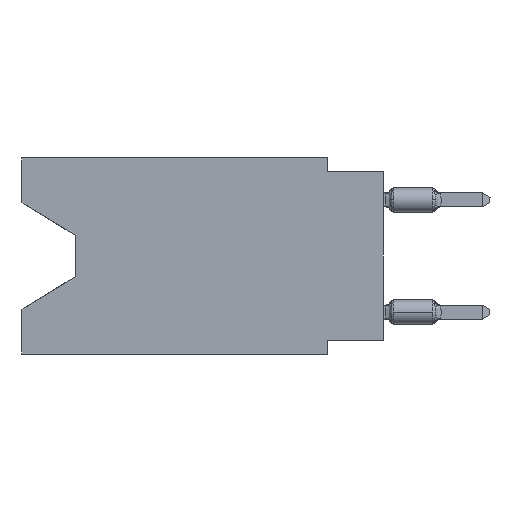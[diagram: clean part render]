
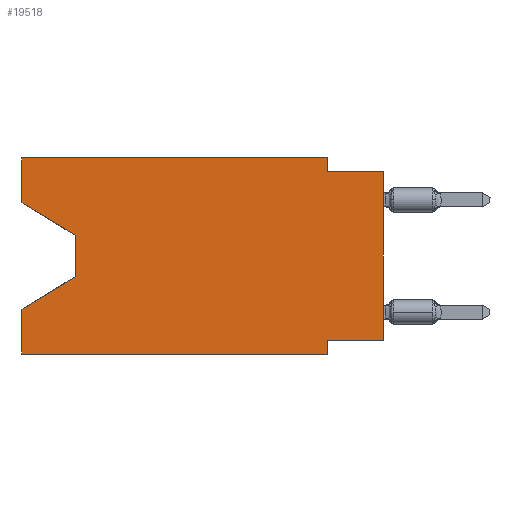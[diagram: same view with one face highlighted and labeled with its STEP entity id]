
A CAD part, left-side view. The second image highlights one B-rep face of the part: STEP entity #19518.
In plain terms, the highlighted planar face has unit normal (-1, 0, 0).
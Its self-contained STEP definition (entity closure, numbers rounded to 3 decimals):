
#23 = CARTESIAN_POINT ( 'NONE',  ( 0., 0., -0.635 ) ) ;
#571 = ORIENTED_EDGE ( 'NONE', *, *, #31390, .T. ) ;
#642 = FACE_OUTER_BOUND ( 'NONE', #12279, .T. ) ;
#667 = LINE ( 'NONE', #24504, #34688 ) ;
#1643 = VECTOR ( 'NONE', #34001, 1000. ) ;
#1932 = EDGE_CURVE ( 'NONE', #30288, #29172, #25603, .T. ) ;
#2011 = CARTESIAN_POINT ( 'NONE',  ( 0., 2.54, -8.255 ) ) ;
#3299 = CARTESIAN_POINT ( 'NONE',  ( 0., 16.383, 0. ) ) ;
#3633 = CARTESIAN_POINT ( 'NONE',  ( 0., 0., -8.255 ) ) ;
#3730 = LINE ( 'NONE', #3299, #38355 ) ;
#4187 = LINE ( 'NONE', #28236, #7925 ) ;
#4588 = CARTESIAN_POINT ( 'NONE',  ( 0., 16.383, -2.038 ) ) ;
#5256 = CARTESIAN_POINT ( 'NONE',  ( 0., 2.54, 0. ) ) ;
#6127 = VECTOR ( 'NONE', #27879, 1000. ) ;
#6147 = EDGE_CURVE ( 'NONE', #29172, #32977, #4187, .T. ) ;
#6573 = LINE ( 'NONE', #20278, #1643 ) ;
#6590 = LINE ( 'NONE', #13998, #31920 ) ;
#6957 = DIRECTION ( 'NONE',  ( 0., 0., -1. ) ) ;
#7413 = DIRECTION ( 'NONE',  ( 0., 0., 1. ) ) ;
#7854 = DIRECTION ( 'NONE',  ( 0., 0., 1. ) ) ;
#7925 = VECTOR ( 'NONE', #41972, 1000. ) ;
#8308 = CARTESIAN_POINT ( 'NONE',  ( 0., 16.383, 0. ) ) ;
#8852 = ORIENTED_EDGE ( 'NONE', *, *, #20858, .T. ) ;
#9142 = VERTEX_POINT ( 'NONE', #43704 ) ;
#9384 = CARTESIAN_POINT ( 'NONE',  ( 0., 16.383, 0. ) ) ;
#9746 = EDGE_CURVE ( 'NONE', #43815, #26328, #14587, .T. ) ;
#9776 = EDGE_CURVE ( 'NONE', #24971, #9142, #38879, .T. ) ;
#10987 = CARTESIAN_POINT ( 'NONE',  ( 0., 16.383, 0. ) ) ;
#11312 = CARTESIAN_POINT ( 'NONE',  ( 0., 13.97, -3.505 ) ) ;
#11656 = CARTESIAN_POINT ( 'NONE',  ( 0., 2.54, 0. ) ) ;
#12279 = EDGE_LOOP ( 'NONE', ( #571, #37443, #8852, #28767, #33993, #18438, #20446, #41958, #36684, #40511, #17150, #42163 ) ) ;
#13998 = CARTESIAN_POINT ( 'NONE',  ( 0., 16.383, -2.038 ) ) ;
#14339 = PLANE ( 'NONE',  #37419 ) ;
#14587 = LINE ( 'NONE', #17315, #6127 ) ;
#16115 = CARTESIAN_POINT ( 'NONE',  ( 0., 2.54, -0.635 ) ) ;
#17145 = VERTEX_POINT ( 'NONE', #9384 ) ;
#17150 = ORIENTED_EDGE ( 'NONE', *, *, #29215, .F. ) ;
#17315 = CARTESIAN_POINT ( 'NONE',  ( 0., 16.383, -8.89 ) ) ;
#18263 = EDGE_CURVE ( 'NONE', #43450, #32977, #21834, .T. ) ;
#18438 = ORIENTED_EDGE ( 'NONE', *, *, #32473, .F. ) ;
#18706 = VERTEX_POINT ( 'NONE', #26655 ) ;
#19518 = ADVANCED_FACE ( 'NONE', ( #642 ), #14339, .F. ) ;
#20212 = DIRECTION ( 'NONE',  ( 1., 0., 0. ) ) ;
#20272 = CARTESIAN_POINT ( 'NONE',  ( 0., 2.54, -8.89 ) ) ;
#20278 = CARTESIAN_POINT ( 'NONE',  ( 0., 13.97, -5.385 ) ) ;
#20446 = ORIENTED_EDGE ( 'NONE', *, *, #37303, .F. ) ;
#20591 = DIRECTION ( 'NONE',  ( 0., 1., 0. ) ) ;
#20858 = EDGE_CURVE ( 'NONE', #9142, #18706, #6573, .T. ) ;
#21834 = LINE ( 'NONE', #31955, #42554 ) ;
#23363 = VECTOR ( 'NONE', #34848, 1000. ) ;
#23472 = CARTESIAN_POINT ( 'NONE',  ( 0., 2.54, -8.89 ) ) ;
#24504 = CARTESIAN_POINT ( 'NONE',  ( 0., 16.383, 0. ) ) ;
#24971 = VERTEX_POINT ( 'NONE', #11312 ) ;
#25371 = DIRECTION ( 'NONE',  ( 0., 0., -1. ) ) ;
#25603 = LINE ( 'NONE', #11656, #36540 ) ;
#26328 = VERTEX_POINT ( 'NONE', #20272 ) ;
#26655 = CARTESIAN_POINT ( 'NONE',  ( 0., 16.383, -6.852 ) ) ;
#26836 = LINE ( 'NONE', #23472, #28388 ) ;
#27544 = LINE ( 'NONE', #37450, #40478 ) ;
#27879 = DIRECTION ( 'NONE',  ( 0., -1., 0. ) ) ;
#28236 = CARTESIAN_POINT ( 'NONE',  ( 0., 0., -0.635 ) ) ;
#28388 = VECTOR ( 'NONE', #40327, 1000. ) ;
#28647 = VERTEX_POINT ( 'NONE', #2011 ) ;
#28767 = ORIENTED_EDGE ( 'NONE', *, *, #41058, .F. ) ;
#29172 = VERTEX_POINT ( 'NONE', #16115 ) ;
#29215 = EDGE_CURVE ( 'NONE', #17145, #30288, #3730, .T. ) ;
#30288 = VERTEX_POINT ( 'NONE', #5256 ) ;
#30413 = DIRECTION ( 'NONE',  ( 0., -0.855, -0.519 ) ) ;
#31254 = CARTESIAN_POINT ( 'NONE',  ( 0., 13.97, -3.505 ) ) ;
#31390 = EDGE_CURVE ( 'NONE', #37545, #24971, #6590, .T. ) ;
#31920 = VECTOR ( 'NONE', #30413, 1000. ) ;
#31955 = CARTESIAN_POINT ( 'NONE',  ( 0., 0., 0. ) ) ;
#32473 = EDGE_CURVE ( 'NONE', #28647, #26328, #26836, .T. ) ;
#32977 = VERTEX_POINT ( 'NONE', #23 ) ;
#33380 = VECTOR ( 'NONE', #7854, 1000. ) ;
#33993 = ORIENTED_EDGE ( 'NONE', *, *, #9746, .T. ) ;
#34001 = DIRECTION ( 'NONE',  ( 0., 0.855, -0.519 ) ) ;
#34688 = VECTOR ( 'NONE', #7413, 1000. ) ;
#34848 = DIRECTION ( 'NONE',  ( 0., 0., -1. ) ) ;
#35559 = DIRECTION ( 'NONE',  ( 0., 0., 1. ) ) ;
#36540 = VECTOR ( 'NONE', #25371, 1000. ) ;
#36684 = ORIENTED_EDGE ( 'NONE', *, *, #6147, .F. ) ;
#37303 = EDGE_CURVE ( 'NONE', #43450, #28647, #27544, .T. ) ;
#37419 = AXIS2_PLACEMENT_3D ( 'NONE', #10987, #20212, #6957 ) ;
#37443 = ORIENTED_EDGE ( 'NONE', *, *, #9776, .T. ) ;
#37450 = CARTESIAN_POINT ( 'NONE',  ( 0., 0., -8.255 ) ) ;
#37545 = VERTEX_POINT ( 'NONE', #4588 ) ;
#37908 = EDGE_CURVE ( 'NONE', #37545, #17145, #42051, .T. ) ;
#38355 = VECTOR ( 'NONE', #40851, 1000. ) ;
#38879 = LINE ( 'NONE', #31254, #23363 ) ;
#40327 = DIRECTION ( 'NONE',  ( 0., 0., -1. ) ) ;
#40473 = CARTESIAN_POINT ( 'NONE',  ( 0., 16.383, -8.89 ) ) ;
#40478 = VECTOR ( 'NONE', #20591, 1000. ) ;
#40511 = ORIENTED_EDGE ( 'NONE', *, *, #1932, .F. ) ;
#40851 = DIRECTION ( 'NONE',  ( 0., -1., 0. ) ) ;
#41058 = EDGE_CURVE ( 'NONE', #43815, #18706, #667, .T. ) ;
#41958 = ORIENTED_EDGE ( 'NONE', *, *, #18263, .T. ) ;
#41972 = DIRECTION ( 'NONE',  ( 0., -1., 0. ) ) ;
#42051 = LINE ( 'NONE', #8308, #33380 ) ;
#42163 = ORIENTED_EDGE ( 'NONE', *, *, #37908, .F. ) ;
#42554 = VECTOR ( 'NONE', #35559, 1000. ) ;
#43450 = VERTEX_POINT ( 'NONE', #3633 ) ;
#43704 = CARTESIAN_POINT ( 'NONE',  ( 0., 13.97, -5.385 ) ) ;
#43815 = VERTEX_POINT ( 'NONE', #40473 ) ;
